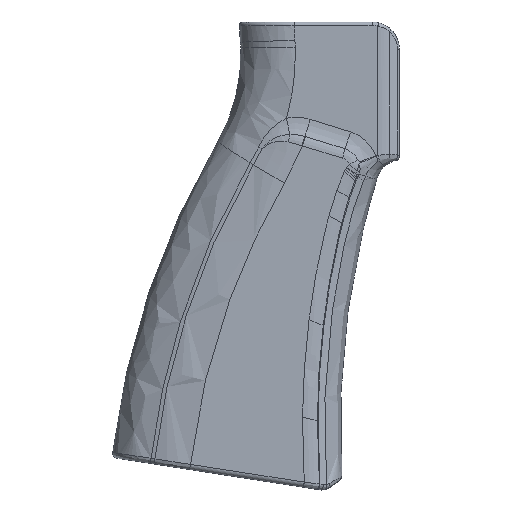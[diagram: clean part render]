
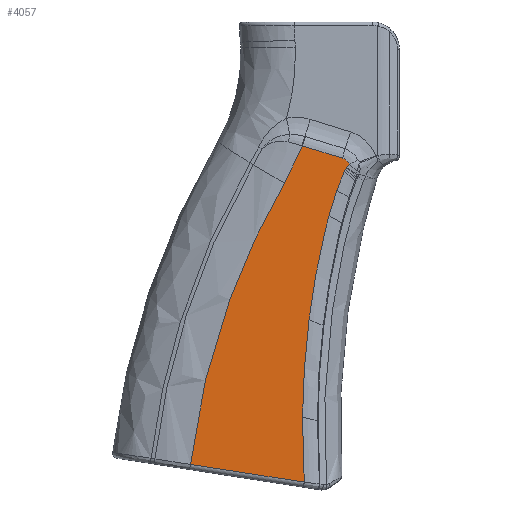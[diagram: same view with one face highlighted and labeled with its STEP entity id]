
A CAD part, left-side view. The second image highlights one B-rep face of the part: STEP entity #4057.
In plain terms, the highlighted planar face has unit normal (-1, 0, 0).
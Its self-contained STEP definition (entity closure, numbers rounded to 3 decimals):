
#412=B_SPLINE_CURVE_WITH_KNOTS('',3,(#10057,#10058,#10059,#10060,#10061),
 .UNSPECIFIED.,.F.,.F.,(4,1,4),(-6.95,-2.981,-0.008),
 .UNSPECIFIED.);
#416=B_SPLINE_CURVE_WITH_KNOTS('',3,(#10097,#10098,#10099,#10100,#10101,
#10102,#10103),.UNSPECIFIED.,.F.,.F.,(4,3,4),(-0.065,0.,1.429),
 .UNSPECIFIED.);
#417=B_SPLINE_CURVE_WITH_KNOTS('',3,(#10105,#10106,#10107,#10108),
 .UNSPECIFIED.,.F.,.F.,(4,4),(1.429,3.664),
 .UNSPECIFIED.);
#418=B_SPLINE_CURVE_WITH_KNOTS('',3,(#10110,#10111,#10112,#10113,#10114,
#10115),.UNSPECIFIED.,.F.,.F.,(4,2,4),(3.664,5.716,
5.716),.UNSPECIFIED.);
#419=B_SPLINE_CURVE_WITH_KNOTS('',3,(#10117,#10118,#10119,#10120),
 .UNSPECIFIED.,.F.,.F.,(4,4),(5.716,6.101),
 .UNSPECIFIED.);
#420=B_SPLINE_CURVE_WITH_KNOTS('',3,(#10122,#10123,#10124,#10125),
 .UNSPECIFIED.,.F.,.F.,(4,4),(6.101,6.711),
 .UNSPECIFIED.);
#421=B_SPLINE_CURVE_WITH_KNOTS('',3,(#10127,#10128,#10129,#10130),
 .UNSPECIFIED.,.F.,.F.,(4,4),(6.711,7.144),
 .UNSPECIFIED.);
#422=B_SPLINE_CURVE_WITH_KNOTS('',3,(#10132,#10133,#10134,#10135),
 .UNSPECIFIED.,.F.,.F.,(4,4),(7.144,7.197),
 .UNSPECIFIED.);
#423=B_SPLINE_CURVE_WITH_KNOTS('',3,(#10137,#10138,#10139,#10140),
 .UNSPECIFIED.,.F.,.F.,(4,4),(7.197,7.255),
 .UNSPECIFIED.);
#424=B_SPLINE_CURVE_WITH_KNOTS('',3,(#10147,#10148,#10149,#10150),
 .UNSPECIFIED.,.F.,.F.,(4,4),(-0.498,0.467),
 .UNSPECIFIED.);
#588=LINE('',#9729,#716);
#590=LINE('',#10142,#718);
#591=LINE('',#10146,#719);
#716=VECTOR('',#5213,10.);
#718=VECTOR('',#5235,10.);
#719=VECTOR('',#5238,10.);
#771=PLANE('',#4451);
#977=FACE_OUTER_BOUND('',#1258,.T.);
#1258=EDGE_LOOP('',(#3457,#3458,#3459,#3460,#3461,#3462,#3463,#3464,#3465,
#3466,#3467,#3468,#3469,#3470));
#1533=CIRCLE('',#4452,2.695);
#1849=VERTEX_POINT('',#9718);
#1851=VERTEX_POINT('',#9727);
#1864=VERTEX_POINT('',#10056);
#1867=VERTEX_POINT('',#10096);
#1868=VERTEX_POINT('',#10104);
#1869=VERTEX_POINT('',#10109);
#1870=VERTEX_POINT('',#10116);
#1871=VERTEX_POINT('',#10121);
#1872=VERTEX_POINT('',#10126);
#1873=VERTEX_POINT('',#10131);
#1874=VERTEX_POINT('',#10136);
#1875=VERTEX_POINT('',#10141);
#1876=VERTEX_POINT('',#10143);
#1877=VERTEX_POINT('',#10145);
#2393=EDGE_CURVE('',#1849,#1851,#588,.T.);
#2416=EDGE_CURVE('',#1851,#1864,#412,.T.);
#2420=EDGE_CURVE('',#1849,#1867,#416,.T.);
#2421=EDGE_CURVE('',#1867,#1868,#417,.T.);
#2422=EDGE_CURVE('',#1868,#1869,#418,.T.);
#2423=EDGE_CURVE('',#1869,#1870,#419,.T.);
#2424=EDGE_CURVE('',#1870,#1871,#420,.T.);
#2425=EDGE_CURVE('',#1871,#1872,#421,.T.);
#2426=EDGE_CURVE('',#1872,#1873,#422,.T.);
#2427=EDGE_CURVE('',#1873,#1874,#423,.T.);
#2428=EDGE_CURVE('',#1875,#1874,#590,.T.);
#2429=EDGE_CURVE('',#1876,#1875,#1533,.T.);
#2430=EDGE_CURVE('',#1877,#1876,#591,.T.);
#2431=EDGE_CURVE('',#1864,#1877,#424,.T.);
#3457=ORIENTED_EDGE('',*,*,#2393,.F.);
#3458=ORIENTED_EDGE('',*,*,#2420,.T.);
#3459=ORIENTED_EDGE('',*,*,#2421,.T.);
#3460=ORIENTED_EDGE('',*,*,#2422,.T.);
#3461=ORIENTED_EDGE('',*,*,#2423,.T.);
#3462=ORIENTED_EDGE('',*,*,#2424,.T.);
#3463=ORIENTED_EDGE('',*,*,#2425,.T.);
#3464=ORIENTED_EDGE('',*,*,#2426,.T.);
#3465=ORIENTED_EDGE('',*,*,#2427,.T.);
#3466=ORIENTED_EDGE('',*,*,#2428,.F.);
#3467=ORIENTED_EDGE('',*,*,#2429,.F.);
#3468=ORIENTED_EDGE('',*,*,#2430,.F.);
#3469=ORIENTED_EDGE('',*,*,#2431,.F.);
#3470=ORIENTED_EDGE('',*,*,#2416,.F.);
#4057=ADVANCED_FACE('',(#977),#771,.T.);
#4451=AXIS2_PLACEMENT_3D('',#10095,#5233,#5234);
#4452=AXIS2_PLACEMENT_3D('',#10144,#5236,#5237);
#5213=DIRECTION('',(0.,0.988,0.154));
#5233=DIRECTION('center_axis',(-1.,0.,0.));
#5234=DIRECTION('ref_axis',(0.,-1.,0.));
#5235=DIRECTION('',(0.,0.65,-0.76));
#5236=DIRECTION('center_axis',(1.,0.,0.));
#5237=DIRECTION('ref_axis',(0.,-0.599,0.801));
#5238=DIRECTION('',(0.,-0.955,-0.296));
#9718=CARTESIAN_POINT('',(-12.74,-132.168,-116.174));
#9727=CARTESIAN_POINT('',(-12.74,-105.732,-112.054));
#9729=CARTESIAN_POINT('',(-12.74,-108.052,-112.415));
#10056=CARTESIAN_POINT('',(-12.74,-127.571,-46.672));
#10057=CARTESIAN_POINT('Ctrl Pts',(-12.74,-105.732,
-112.054));
#10058=CARTESIAN_POINT('Ctrl Pts',(-12.74,-107.286,-98.917));
#10059=CARTESIAN_POINT('Ctrl Pts',(-12.74,-112.706,-76.259));
#10060=CARTESIAN_POINT('Ctrl Pts',(-12.74,-122.587,
-55.237));
#10061=CARTESIAN_POINT('Ctrl Pts',(-12.74,-127.571,
-46.672));
#10095=CARTESIAN_POINT('Origin',(-12.74,-124.662,-63.494));
#10096=CARTESIAN_POINT('',(-12.74,-131.769,-101.065));
#10097=CARTESIAN_POINT('Ctrl Pts',(-12.74,-132.168,-116.174));
#10098=CARTESIAN_POINT('Ctrl Pts',(-12.74,-132.154,-115.954));
#10099=CARTESIAN_POINT('Ctrl Pts',(-12.74,-132.141,-115.733));
#10100=CARTESIAN_POINT('Ctrl Pts',(-12.74,-132.127,-115.513));
#10101=CARTESIAN_POINT('Ctrl Pts',(-12.74,-131.837,
-110.702));
#10102=CARTESIAN_POINT('Ctrl Pts',(-12.74,-131.717,
-105.883));
#10103=CARTESIAN_POINT('Ctrl Pts',(-12.74,-131.769,-101.065));
#10104=CARTESIAN_POINT('',(-12.74,-133.268,-78.508));
#10105=CARTESIAN_POINT('Ctrl Pts',(-12.74,-131.769,-101.065));
#10106=CARTESIAN_POINT('Ctrl Pts',(-12.74,-131.849,
-93.527));
#10107=CARTESIAN_POINT('Ctrl Pts',(-12.74,-132.345,
-85.993));
#10108=CARTESIAN_POINT('Ctrl Pts',(-12.74,-133.268,-78.508));
#10109=CARTESIAN_POINT('',(-12.74,-136.957,-58.071));
#10110=CARTESIAN_POINT('Ctrl Pts',(-12.74,-133.268,-78.508));
#10111=CARTESIAN_POINT('Ctrl Pts',(-12.74,-134.115,
-71.642));
#10112=CARTESIAN_POINT('Ctrl Pts',(-12.74,-135.322,
-64.81));
#10113=CARTESIAN_POINT('Ctrl Pts',(-12.74,-136.957,
-58.071));
#10114=CARTESIAN_POINT('Ctrl Pts',(-12.74,-136.957,
-58.071));
#10115=CARTESIAN_POINT('Ctrl Pts',(-12.74,-136.957,
-58.071));
#10116=CARTESIAN_POINT('',(-12.74,-137.929,-54.279));
#10117=CARTESIAN_POINT('Ctrl Pts',(-12.74,-136.957,
-58.071));
#10118=CARTESIAN_POINT('Ctrl Pts',(-12.74,-137.265,
-56.804));
#10119=CARTESIAN_POINT('Ctrl Pts',(-12.74,-137.588,
-55.54));
#10120=CARTESIAN_POINT('Ctrl Pts',(-12.74,-137.929,
-54.279));
#10121=CARTESIAN_POINT('',(-12.74,-139.743,-48.299));
#10122=CARTESIAN_POINT('Ctrl Pts',(-12.74,-137.929,
-54.279));
#10123=CARTESIAN_POINT('Ctrl Pts',(-12.74,-138.466,
-52.289));
#10124=CARTESIAN_POINT('Ctrl Pts',(-12.74,-139.051,
-50.286));
#10125=CARTESIAN_POINT('Ctrl Pts',(-12.74,-139.743,
-48.299));
#10126=CARTESIAN_POINT('',(-12.74,-141.488,-44.063));
#10127=CARTESIAN_POINT('Ctrl Pts',(-12.74,-139.743,
-48.299));
#10128=CARTESIAN_POINT('Ctrl Pts',(-12.74,-140.236,-46.885));
#10129=CARTESIAN_POINT('Ctrl Pts',(-12.74,-140.797,
-45.456));
#10130=CARTESIAN_POINT('Ctrl Pts',(-12.74,-141.488,
-44.063));
#10131=CARTESIAN_POINT('',(-12.74,-141.744,-43.559));
#10132=CARTESIAN_POINT('Ctrl Pts',(-12.74,-141.488,
-44.063));
#10133=CARTESIAN_POINT('Ctrl Pts',(-12.74,-141.572,-43.893));
#10134=CARTESIAN_POINT('Ctrl Pts',(-12.74,-141.658,-43.725));
#10135=CARTESIAN_POINT('Ctrl Pts',(-12.74,-141.744,
-43.559));
#10136=CARTESIAN_POINT('',(-12.74,-142.034,-43.013));
#10137=CARTESIAN_POINT('Ctrl Pts',(-12.74,-141.744,
-43.559));
#10138=CARTESIAN_POINT('Ctrl Pts',(-12.74,-141.838,
-43.377));
#10139=CARTESIAN_POINT('Ctrl Pts',(-12.74,-141.935,
-43.194));
#10140=CARTESIAN_POINT('Ctrl Pts',(-12.74,-142.034,
-43.013));
#10141=CARTESIAN_POINT('',(-12.74,-142.662,-42.278));
#10142=CARTESIAN_POINT('',(-12.74,-142.034,-43.013));
#10143=CARTESIAN_POINT('',(-12.74,-141.03,-40.869));
#10144=CARTESIAN_POINT('Origin',(-12.74,-140.232,-43.443));
#10145=CARTESIAN_POINT('',(-12.74,-131.783,-38.004));
#10146=CARTESIAN_POINT('',(-12.74,-153.895,-44.857));
#10147=CARTESIAN_POINT('Ctrl Pts',(-12.74,-127.571,
-46.672));
#10148=CARTESIAN_POINT('Ctrl Pts',(-12.74,-129.211,
-43.905));
#10149=CARTESIAN_POINT('Ctrl Pts',(-12.74,-130.621,
-41.003));
#10150=CARTESIAN_POINT('Ctrl Pts',(-12.74,-131.783,
-38.004));
